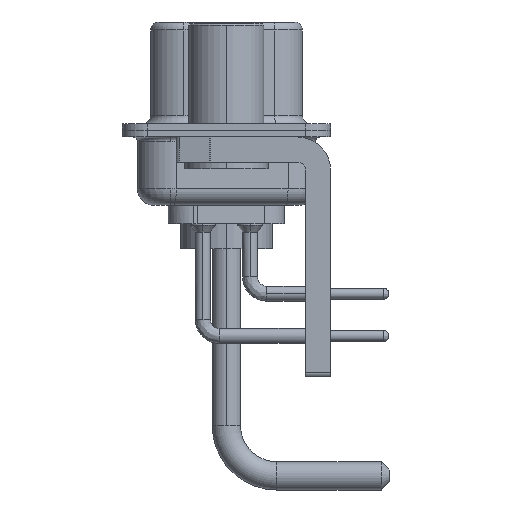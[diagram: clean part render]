
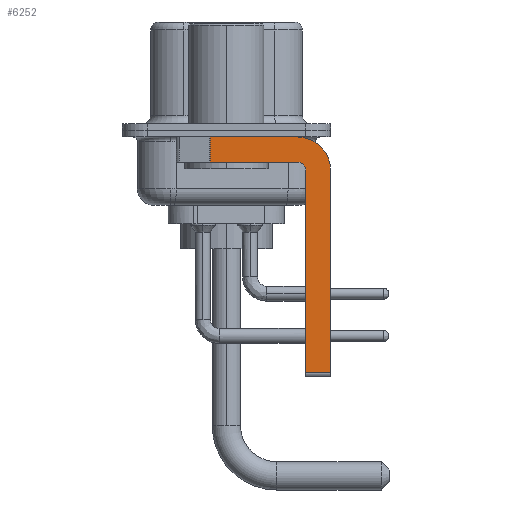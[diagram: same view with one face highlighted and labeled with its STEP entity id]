
A CAD part, left-side view. The second image highlights one B-rep face of the part: STEP entity #6252.
In plain terms, the highlighted planar face has unit normal (-1, 0, 0).
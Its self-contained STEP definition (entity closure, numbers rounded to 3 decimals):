
#847 = ORIENTED_EDGE ( 'NONE', *, *, #21295, .F. ) ;
#950 = DIRECTION ( 'NONE',  ( 0., 0., 1. ) ) ;
#978 = CARTESIAN_POINT ( 'NONE',  ( -2.9, -6.25, -14.55 ) ) ;
#1011 = EDGE_CURVE ( 'NONE', #6068, #18395, #15636, .T. ) ;
#1224 = DIRECTION ( 'NONE',  ( -1., 0., 0. ) ) ;
#2830 = DIRECTION ( 'NONE',  ( 0., -1., 0. ) ) ;
#2914 = EDGE_CURVE ( 'NONE', #11634, #26109, #8178, .T. ) ;
#3440 = LINE ( 'NONE', #12501, #16017 ) ;
#3766 = CARTESIAN_POINT ( 'NONE',  ( -2.9, -6.25, -2.4 ) ) ;
#5080 = CARTESIAN_POINT ( 'NONE',  ( -2.9, -4.25, -0.4 ) ) ;
#5130 = DIRECTION ( 'NONE',  ( 1., 0., 0. ) ) ;
#5168 = EDGE_CURVE ( 'NONE', #22757, #15678, #6104, .T. ) ;
#6068 = VERTEX_POINT ( 'NONE', #25838 ) ;
#6104 = LINE ( 'NONE', #18785, #26524 ) ;
#6252 = ADVANCED_FACE ( 'NONE', ( #22236 ), #9180, .F. ) ;
#6388 = CIRCLE ( 'NONE', #14664, 0.5 ) ;
#6965 = VECTOR ( 'NONE', #25763, 1000. ) ;
#7100 = VERTEX_POINT ( 'NONE', #22003 ) ;
#7672 = ORIENTED_EDGE ( 'NONE', *, *, #20233, .F. ) ;
#7830 = LINE ( 'NONE', #18902, #24080 ) ;
#8178 = LINE ( 'NONE', #12492, #10257 ) ;
#9051 = EDGE_CURVE ( 'NONE', #22757, #26109, #7830, .T. ) ;
#9180 = PLANE ( 'NONE',  #23658 ) ;
#10257 = VECTOR ( 'NONE', #10329, 1000. ) ;
#10329 = DIRECTION ( 'NONE',  ( 0., 1., 0. ) ) ;
#11102 = CARTESIAN_POINT ( 'NONE',  ( -2.9, -4.25, -2.4 ) ) ;
#11634 = VERTEX_POINT ( 'NONE', #20027 ) ;
#11853 = EDGE_CURVE ( 'NONE', #6068, #7100, #23880, .T. ) ;
#11887 = AXIS2_PLACEMENT_3D ( 'NONE', #11102, #13537, #15985 ) ;
#12492 = CARTESIAN_POINT ( 'NONE',  ( -2.9, -4.25, -1.9 ) ) ;
#12501 = CARTESIAN_POINT ( 'NONE',  ( -2.9, -6.25, -2.4 ) ) ;
#13295 = CARTESIAN_POINT ( 'NONE',  ( -2.9, 0.978, -0.4 ) ) ;
#13301 = ORIENTED_EDGE ( 'NONE', *, *, #9051, .T. ) ;
#13537 = DIRECTION ( 'NONE',  ( 1., 0., 0. ) ) ;
#14223 = ORIENTED_EDGE ( 'NONE', *, *, #1011, .T. ) ;
#14557 = CARTESIAN_POINT ( 'NONE',  ( -2.9, -4.75, -14.8 ) ) ;
#14664 = AXIS2_PLACEMENT_3D ( 'NONE', #25081, #1224, #950 ) ;
#15636 = LINE ( 'NONE', #17935, #22828 ) ;
#15678 = VERTEX_POINT ( 'NONE', #5080 ) ;
#15963 = VERTEX_POINT ( 'NONE', #3766 ) ;
#15985 = DIRECTION ( 'NONE',  ( 0., 0., -1. ) ) ;
#16017 = VECTOR ( 'NONE', #23265, 1000. ) ;
#16218 = ORIENTED_EDGE ( 'NONE', *, *, #5168, .F. ) ;
#16482 = DIRECTION ( 'NONE',  ( 0., 0., -1. ) ) ;
#17935 = CARTESIAN_POINT ( 'NONE',  ( -2.9, -4.25, -14.55 ) ) ;
#18395 = VERTEX_POINT ( 'NONE', #978 ) ;
#18785 = CARTESIAN_POINT ( 'NONE',  ( -2.9, 3., -0.4 ) ) ;
#18902 = CARTESIAN_POINT ( 'NONE',  ( -2.9, 0.978, -1.9 ) ) ;
#19585 = ORIENTED_EDGE ( 'NONE', *, *, #25839, .F. ) ;
#20027 = CARTESIAN_POINT ( 'NONE',  ( -2.9, -4.25, -1.9 ) ) ;
#20233 = EDGE_CURVE ( 'NONE', #7100, #11634, #6388, .T. ) ;
#21295 = EDGE_CURVE ( 'NONE', #15963, #18395, #3440, .T. ) ;
#21512 = CIRCLE ( 'NONE', #11887, 2. ) ;
#22003 = CARTESIAN_POINT ( 'NONE',  ( -2.9, -4.75, -2.4 ) ) ;
#22236 = FACE_OUTER_BOUND ( 'NONE', #25636, .T. ) ;
#22757 = VERTEX_POINT ( 'NONE', #13295 ) ;
#22828 = VECTOR ( 'NONE', #2830, 1000. ) ;
#22948 = DIRECTION ( 'NONE',  ( 0., 0., -1. ) ) ;
#23265 = DIRECTION ( 'NONE',  ( 0., 0., -1. ) ) ;
#23658 = AXIS2_PLACEMENT_3D ( 'NONE', #26691, #5130, #22948 ) ;
#23880 = LINE ( 'NONE', #14557, #6965 ) ;
#24080 = VECTOR ( 'NONE', #16482, 1000. ) ;
#24549 = ORIENTED_EDGE ( 'NONE', *, *, #11853, .F. ) ;
#25081 = CARTESIAN_POINT ( 'NONE',  ( -2.9, -4.25, -2.4 ) ) ;
#25636 = EDGE_LOOP ( 'NONE', ( #16218, #13301, #27179, #7672, #24549, #14223, #847, #19585 ) ) ;
#25672 = DIRECTION ( 'NONE',  ( 0., -1., 0. ) ) ;
#25763 = DIRECTION ( 'NONE',  ( 0., 0., 1. ) ) ;
#25839 = EDGE_CURVE ( 'NONE', #15678, #15963, #21512, .T. ) ;
#25838 = CARTESIAN_POINT ( 'NONE',  ( -2.9, -4.75, -14.55 ) ) ;
#26109 = VERTEX_POINT ( 'NONE', #27728 ) ;
#26524 = VECTOR ( 'NONE', #25672, 1000. ) ;
#26691 = CARTESIAN_POINT ( 'NONE',  ( -2.9, -4.25, -2.4 ) ) ;
#27179 = ORIENTED_EDGE ( 'NONE', *, *, #2914, .F. ) ;
#27728 = CARTESIAN_POINT ( 'NONE',  ( -2.9, 0.978, -1.9 ) ) ;
